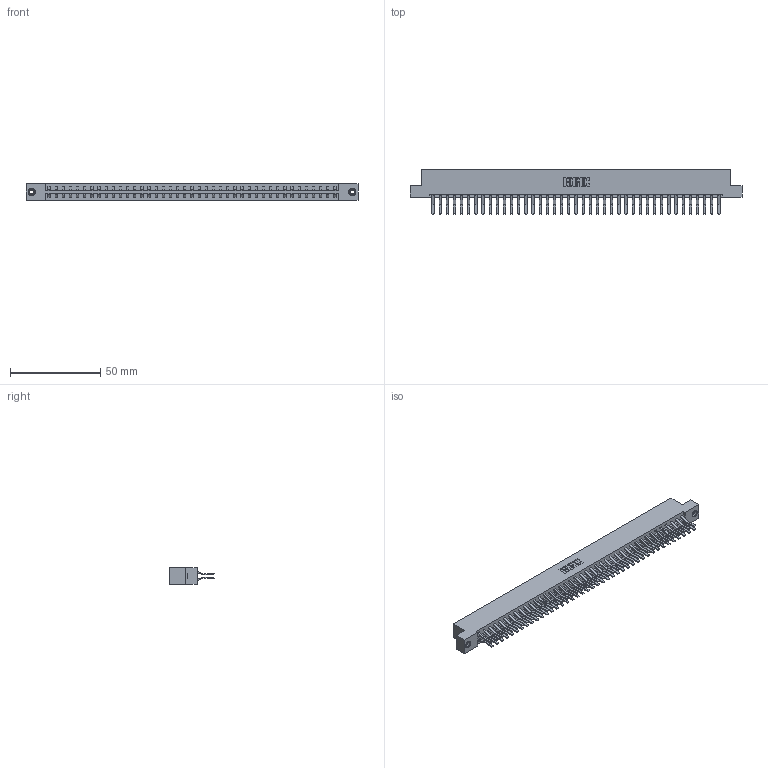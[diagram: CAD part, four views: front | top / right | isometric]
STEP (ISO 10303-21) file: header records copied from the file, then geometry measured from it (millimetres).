
FILE_DESCRIPTION (( 'STEP AP203' ), '1' );
FILE_NAME ('833-082-560-208.STEP', '2020-06-06T00:36:39', ( '' ), ( '' ), 'SwSTEP 2.0', 'SolidWorks 2020', '' );
FILE_SCHEMA (( 'CONFIG_CONTROL_DESIGN' ));
Length unit declared in the file: inch
Products named in the file (4): 833-082-560-208; 833 Part_Flush - .156 Dia - TI; 345-250-001_345-250-003-102; 345-292-001_560 Tail
Assembly tree (85 placements, depth 2):
  833-082-560-208
    833 Part_Flush - .156 Dia - TI
    345-292-001_560 Tail  x82
    345-250-001_345-250-003-102  x2
Bounding box: 184 x 24.78 x 9.4 mm (x, y, z)
Volume: 19306.7 mm3; surface area: 24369.6 mm2
Topology: 85 solids, 85 shells, 4602 faces, 13649 edges, 8982 vertices
Faces by surface type: plane 3054, cylinder 1532, cone 12, torus 4
Entity records: 27780 total; most frequent: CARTESIAN_POINT 4589, ORIENTED_EDGE 4518, DIRECTION 3957, EDGE_CURVE 2259, LINE 2107, VECTOR 2107, VERTEX_POINT 1500, AXIS2_PLACEMENT_3D 925
